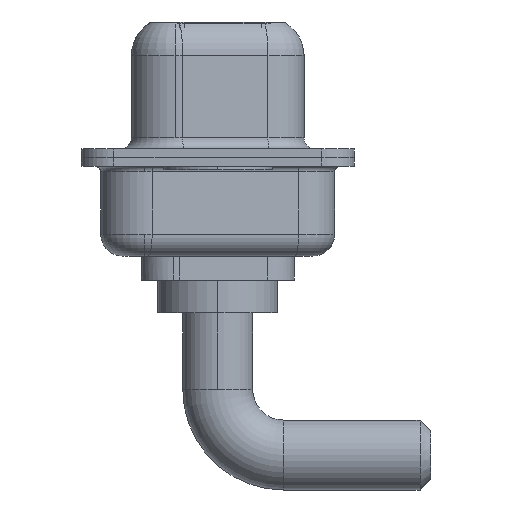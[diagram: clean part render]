
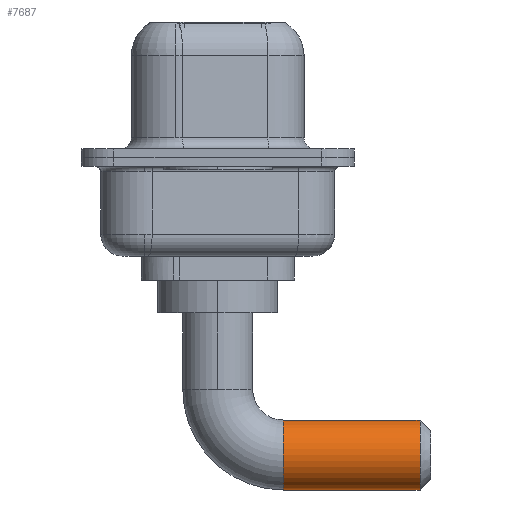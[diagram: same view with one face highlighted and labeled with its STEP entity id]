
A CAD part, left-side view. The second image highlights one B-rep face of the part: STEP entity #7687.
In plain terms, the highlighted cylindrical face has radius 1.6 mm (diameter 3.2 mm), a partial arc.
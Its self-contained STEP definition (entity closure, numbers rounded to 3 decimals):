
#75 = EDGE_CURVE ( 'NONE', #7125, #3015, #9864, .T. ) ;
#563 = FACE_OUTER_BOUND ( 'NONE', #9598, .T. ) ;
#568 = EDGE_CURVE ( 'NONE', #3015, #7920, #8792, .T. ) ;
#654 = EDGE_CURVE ( 'NONE', #7920, #2792, #7664, .T. ) ;
#837 = DIRECTION ( 'NONE',  ( 0., -1., 0. ) ) ;
#1306 = ORIENTED_EDGE ( 'NONE', *, *, #654, .T. ) ;
#2327 = CARTESIAN_POINT ( 'NONE',  ( 0., -3., -6.5 ) ) ;
#2494 = AXIS2_PLACEMENT_3D ( 'NONE', #10586, #7971, #5263 ) ;
#2792 = VERTEX_POINT ( 'NONE', #9899 ) ;
#3015 = VERTEX_POINT ( 'NONE', #8624 ) ;
#3523 = VECTOR ( 'NONE', #9976, 1000. ) ;
#5000 = DIRECTION ( 'NONE',  ( 0., -1., 0. ) ) ;
#5097 = ORIENTED_EDGE ( 'NONE', *, *, #568, .T. ) ;
#5106 = AXIS2_PLACEMENT_3D ( 'NONE', #2327, #5000, #8182 ) ;
#5263 = DIRECTION ( 'NONE',  ( 0., 0., -1. ) ) ;
#5530 = CARTESIAN_POINT ( 'NONE',  ( 0., -3., -4.9 ) ) ;
#5645 = CARTESIAN_POINT ( 'NONE',  ( 0., -3., -4.9 ) ) ;
#5889 = EDGE_CURVE ( 'NONE', #7125, #2792, #10856, .T. ) ;
#5991 = ORIENTED_EDGE ( 'NONE', *, *, #75, .T. ) ;
#6555 = VECTOR ( 'NONE', #837, 1000. ) ;
#6862 = ORIENTED_EDGE ( 'NONE', *, *, #5889, .F. ) ;
#6869 = CARTESIAN_POINT ( 'NONE',  ( 0., -3., -8.1 ) ) ;
#7125 = VERTEX_POINT ( 'NONE', #5530 ) ;
#7664 = CIRCLE ( 'NONE', #2494, 1.6 ) ;
#7687 = ADVANCED_FACE ( 'NONE', ( #563 ), #11128, .T. ) ;
#7920 = VERTEX_POINT ( 'NONE', #10580 ) ;
#7971 = DIRECTION ( 'NONE',  ( 0., 1., 0. ) ) ;
#8182 = DIRECTION ( 'NONE',  ( 0., 0., -1. ) ) ;
#8624 = CARTESIAN_POINT ( 'NONE',  ( 0., -3., -8.1 ) ) ;
#8635 = CARTESIAN_POINT ( 'NONE',  ( 0., -3., -6.5 ) ) ;
#8792 = LINE ( 'NONE', #6869, #6555 ) ;
#9598 = EDGE_LOOP ( 'NONE', ( #6862, #5991, #5097, #1306 ) ) ;
#9864 = CIRCLE ( 'NONE', #10427, 1.6 ) ;
#9899 = CARTESIAN_POINT ( 'NONE',  ( 0., -9.25, -4.9 ) ) ;
#9976 = DIRECTION ( 'NONE',  ( 0., -1., 0. ) ) ;
#10420 = DIRECTION ( 'NONE',  ( 0., -1., 0. ) ) ;
#10427 = AXIS2_PLACEMENT_3D ( 'NONE', #8635, #10420, #11478 ) ;
#10580 = CARTESIAN_POINT ( 'NONE',  ( 0., -9.25, -8.1 ) ) ;
#10586 = CARTESIAN_POINT ( 'NONE',  ( 0., -9.25, -6.5 ) ) ;
#10856 = LINE ( 'NONE', #5645, #3523 ) ;
#11128 = CYLINDRICAL_SURFACE ( 'NONE', #5106, 1.6 ) ;
#11478 = DIRECTION ( 'NONE',  ( -1., 0., 0. ) ) ;
